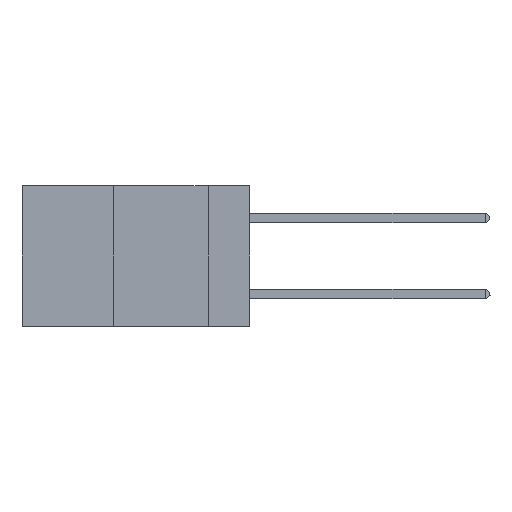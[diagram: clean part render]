
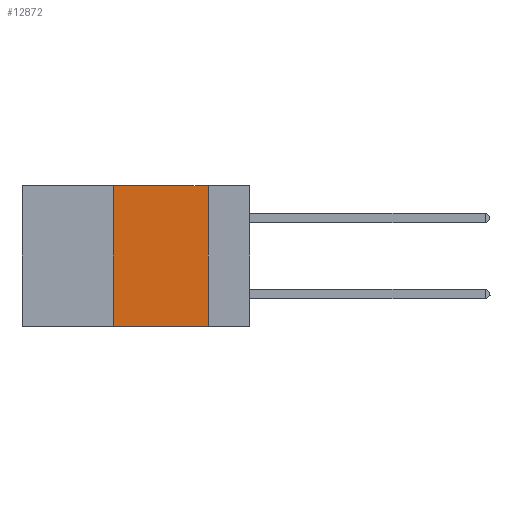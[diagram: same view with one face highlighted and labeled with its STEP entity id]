
A CAD part, left-side view. The second image highlights one B-rep face of the part: STEP entity #12872.
In plain terms, the highlighted planar face has unit normal (-1, 0, 0).
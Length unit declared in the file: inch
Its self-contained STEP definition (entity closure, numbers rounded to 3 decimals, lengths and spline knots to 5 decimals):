
#228 = EDGE_CURVE ( 'NONE', #16732, #16513, #18910, .T. ) ;
#2890 = DIRECTION ( 'NONE',  ( 0., 0., 1. ) ) ;
#3826 = CARTESIAN_POINT ( 'NONE',  ( 0., 0.11, 0. ) ) ;
#5323 = DIRECTION ( 'NONE',  ( 0., -1., 0. ) ) ;
#5334 = DIRECTION ( 'NONE',  ( 1., 0., 0. ) ) ;
#5362 = DIRECTION ( 'NONE',  ( 0., 0., -1. ) ) ;
#5652 = VECTOR ( 'NONE', #15218, 39.37008 ) ;
#6639 = EDGE_CURVE ( 'NONE', #13968, #16732, #16842, .T. ) ;
#7216 = LINE ( 'NONE', #19197, #14933 ) ;
#7448 = VECTOR ( 'NONE', #5362, 39.37008 ) ;
#7598 = CARTESIAN_POINT ( 'NONE',  ( 0., 0.11, 0. ) ) ;
#8074 = FACE_OUTER_BOUND ( 'NONE', #15283, .T. ) ;
#8189 = VECTOR ( 'NONE', #2890, 39.37008 ) ;
#11436 = CARTESIAN_POINT ( 'NONE',  ( 0., 0.36, 0. ) ) ;
#11508 = PLANE ( 'NONE',  #14991 ) ;
#12872 = ADVANCED_FACE ( 'NONE', ( #8074 ), #11508, .F. ) ;
#13968 = VERTEX_POINT ( 'NONE', #17102 ) ;
#14536 = CARTESIAN_POINT ( 'NONE',  ( 0., 0.11, -0.37 ) ) ;
#14589 = CARTESIAN_POINT ( 'NONE',  ( 0., 0.6, 0. ) ) ;
#14921 = EDGE_CURVE ( 'NONE', #13968, #19289, #7216, .T. ) ;
#14933 = VECTOR ( 'NONE', #5323, 39.37008 ) ;
#14991 = AXIS2_PLACEMENT_3D ( 'NONE', #14589, #5334, #16137 ) ;
#15218 = DIRECTION ( 'NONE',  ( 0., -1., 0. ) ) ;
#15283 = EDGE_LOOP ( 'NONE', ( #15323, #15396, #15496, #15526 ) ) ;
#15323 = ORIENTED_EDGE ( 'NONE', *, *, #15580, .F. ) ;
#15396 = ORIENTED_EDGE ( 'NONE', *, *, #228, .F. ) ;
#15496 = ORIENTED_EDGE ( 'NONE', *, *, #6639, .F. ) ;
#15526 = ORIENTED_EDGE ( 'NONE', *, *, #14921, .T. ) ;
#15580 = EDGE_CURVE ( 'NONE', #16513, #19289, #19702, .T. ) ;
#16137 = DIRECTION ( 'NONE',  ( 0., 0., -1. ) ) ;
#16513 = VERTEX_POINT ( 'NONE', #7598 ) ;
#16732 = VERTEX_POINT ( 'NONE', #11436 ) ;
#16842 = LINE ( 'NONE', #19762, #8189 ) ;
#17102 = CARTESIAN_POINT ( 'NONE',  ( 0., 0.36, -0.37 ) ) ;
#18376 = CARTESIAN_POINT ( 'NONE',  ( 0., 0.6, 0. ) ) ;
#18910 = LINE ( 'NONE', #18376, #5652 ) ;
#19197 = CARTESIAN_POINT ( 'NONE',  ( 0., 0.6, -0.37 ) ) ;
#19289 = VERTEX_POINT ( 'NONE', #14536 ) ;
#19702 = LINE ( 'NONE', #3826, #7448 ) ;
#19762 = CARTESIAN_POINT ( 'NONE',  ( 0., 0.36, 0. ) ) ;
